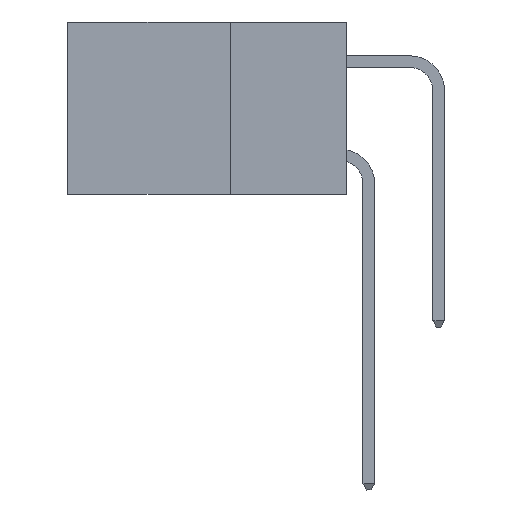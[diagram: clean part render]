
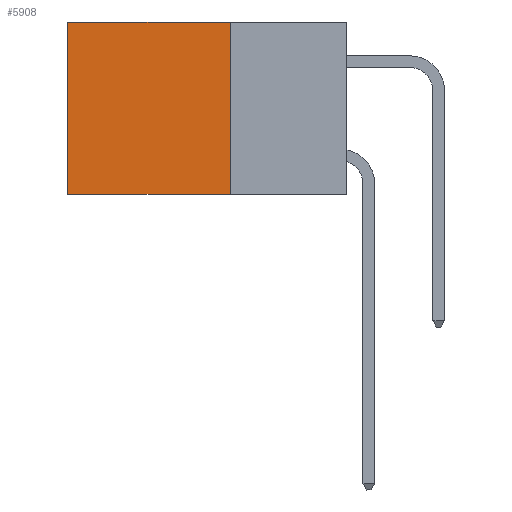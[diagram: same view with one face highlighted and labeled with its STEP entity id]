
A CAD part, left-side view. The second image highlights one B-rep face of the part: STEP entity #5908.
In plain terms, the highlighted planar face has unit normal (-1, 0, 0).
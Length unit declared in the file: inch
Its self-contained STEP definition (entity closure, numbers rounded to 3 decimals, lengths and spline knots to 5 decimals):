
#283 = VECTOR ( 'NONE', #10096, 39.37008 ) ;
#691 = CARTESIAN_POINT ( 'NONE',  ( 0.2875, 0.6, 0. ) ) ;
#1099 = EDGE_CURVE ( 'NONE', #5727, #6019, #3720, .T. ) ;
#1718 = DIRECTION ( 'NONE',  ( 0., 0., -1. ) ) ;
#1730 = DIRECTION ( 'NONE',  ( 1., 0., 0. ) ) ;
#1734 = CARTESIAN_POINT ( 'NONE',  ( 0.2875, 0.25, 0. ) ) ;
#1957 = DIRECTION ( 'NONE',  ( 0., 1., 0. ) ) ;
#2024 = DIRECTION ( 'NONE',  ( 0., 0., -1. ) ) ;
#2045 = PLANE ( 'NONE',  #4906 ) ;
#2058 = FACE_OUTER_BOUND ( 'NONE', #6462, .T. ) ;
#2370 = CARTESIAN_POINT ( 'NONE',  ( 0.2875, 0.25, 0. ) ) ;
#3153 = CARTESIAN_POINT ( 'NONE',  ( 0.2875, 0.6, -0.37 ) ) ;
#3720 = LINE ( 'NONE', #9100, #5569 ) ;
#3761 = CARTESIAN_POINT ( 'NONE',  ( 0.2875, 0.25, 0. ) ) ;
#3811 = EDGE_CURVE ( 'NONE', #5727, #10314, #5215, .T. ) ;
#3977 = DIRECTION ( 'NONE',  ( 0., 0., -1. ) ) ;
#4310 = VECTOR ( 'NONE', #3977, 39.37008 ) ;
#4594 = LINE ( 'NONE', #6653, #4310 ) ;
#4906 = AXIS2_PLACEMENT_3D ( 'NONE', #1734, #1730, #1718 ) ;
#5215 = LINE ( 'NONE', #2370, #9728 ) ;
#5569 = VECTOR ( 'NONE', #1957, 39.37008 ) ;
#5727 = VERTEX_POINT ( 'NONE', #3761 ) ;
#5908 = ADVANCED_FACE ( 'NONE', ( #2058 ), #2045, .F. ) ;
#6019 = VERTEX_POINT ( 'NONE', #691 ) ;
#6462 = EDGE_LOOP ( 'NONE', ( #8915, #11289, #6806, #7079 ) ) ;
#6653 = CARTESIAN_POINT ( 'NONE',  ( 0.2875, 0.6, 0. ) ) ;
#6806 = ORIENTED_EDGE ( 'NONE', *, *, #3811, .F. ) ;
#7079 = ORIENTED_EDGE ( 'NONE', *, *, #1099, .T. ) ;
#7672 = LINE ( 'NONE', #10997, #283 ) ;
#8915 = ORIENTED_EDGE ( 'NONE', *, *, #9099, .T. ) ;
#9099 = EDGE_CURVE ( 'NONE', #6019, #9145, #4594, .T. ) ;
#9100 = CARTESIAN_POINT ( 'NONE',  ( 0.2875, 0.25, 0. ) ) ;
#9145 = VERTEX_POINT ( 'NONE', #3153 ) ;
#9712 = EDGE_CURVE ( 'NONE', #10314, #9145, #7672, .T. ) ;
#9728 = VECTOR ( 'NONE', #2024, 39.37008 ) ;
#10096 = DIRECTION ( 'NONE',  ( 0., 1., 0. ) ) ;
#10314 = VERTEX_POINT ( 'NONE', #10804 ) ;
#10804 = CARTESIAN_POINT ( 'NONE',  ( 0.2875, 0.25, -0.37 ) ) ;
#10997 = CARTESIAN_POINT ( 'NONE',  ( 0.2875, 0.25, -0.37 ) ) ;
#11289 = ORIENTED_EDGE ( 'NONE', *, *, #9712, .F. ) ;
